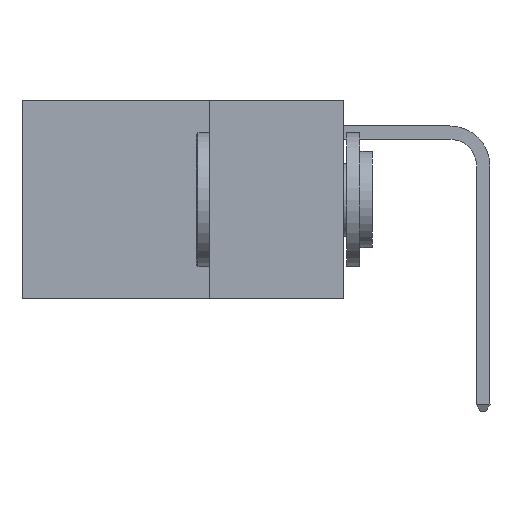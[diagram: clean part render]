
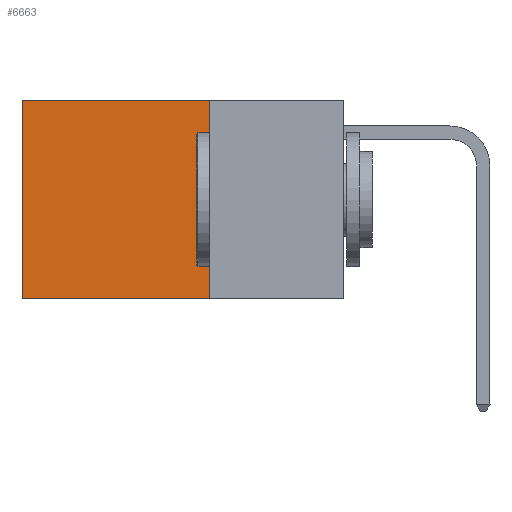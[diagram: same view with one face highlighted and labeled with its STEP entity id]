
A CAD part, left-side view. The second image highlights one B-rep face of the part: STEP entity #6663.
In plain terms, the highlighted planar face has unit normal (-1, 0, 0).
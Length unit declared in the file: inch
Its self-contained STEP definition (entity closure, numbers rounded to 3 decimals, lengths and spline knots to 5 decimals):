
#98 = LINE ( 'NONE', #18927, #11334 ) ;
#818 = CARTESIAN_POINT ( 'NONE',  ( 0.2625, 0.25, 0. ) ) ;
#1428 = EDGE_LOOP ( 'NONE', ( #16039, #3002, #7451, #16599 ) ) ;
#1531 = CARTESIAN_POINT ( 'NONE',  ( 0.2625, 0.6, -0.37 ) ) ;
#1588 = DIRECTION ( 'NONE',  ( 0., 1., 0. ) ) ;
#1598 = DIRECTION ( 'NONE',  ( 0., 0., -1. ) ) ;
#1972 = CARTESIAN_POINT ( 'NONE',  ( 0.2625, 0.6, 0. ) ) ;
#2397 = CARTESIAN_POINT ( 'NONE',  ( 0.2625, 0.6, 0. ) ) ;
#2814 = VERTEX_POINT ( 'NONE', #1531 ) ;
#2885 = DIRECTION ( 'NONE',  ( 0., 1., 0. ) ) ;
#3002 = ORIENTED_EDGE ( 'NONE', *, *, #4521, .F. ) ;
#3308 = LINE ( 'NONE', #9067, #15841 ) ;
#4463 = CARTESIAN_POINT ( 'NONE',  ( 0.2625, 0.25, -0.37 ) ) ;
#4521 = EDGE_CURVE ( 'NONE', #5329, #2814, #98, .T. ) ;
#5253 = DIRECTION ( 'NONE',  ( 0., 0., -1. ) ) ;
#5329 = VERTEX_POINT ( 'NONE', #4463 ) ;
#6663 = ADVANCED_FACE ( 'NONE', ( #7265 ), #14650, .F. ) ;
#6981 = VERTEX_POINT ( 'NONE', #818 ) ;
#7265 = FACE_OUTER_BOUND ( 'NONE', #1428, .T. ) ;
#7451 = ORIENTED_EDGE ( 'NONE', *, *, #9723, .F. ) ;
#9067 = CARTESIAN_POINT ( 'NONE',  ( 0.2625, 0.25, 0. ) ) ;
#9491 = LINE ( 'NONE', #18412, #13895 ) ;
#9723 = EDGE_CURVE ( 'NONE', #6981, #5329, #9491, .T. ) ;
#11334 = VECTOR ( 'NONE', #2885, 39.37008 ) ;
#11668 = CARTESIAN_POINT ( 'NONE',  ( 0.2625, 0.25, 0. ) ) ;
#13013 = DIRECTION ( 'NONE',  ( 1., 0., 0. ) ) ;
#13579 = EDGE_CURVE ( 'NONE', #6981, #14648, #3308, .T. ) ;
#13657 = DIRECTION ( 'NONE',  ( 0., 0., -1. ) ) ;
#13895 = VECTOR ( 'NONE', #5253, 39.37008 ) ;
#14371 = VECTOR ( 'NONE', #13657, 39.37008 ) ;
#14648 = VERTEX_POINT ( 'NONE', #2397 ) ;
#14650 = PLANE ( 'NONE',  #15455 ) ;
#15107 = LINE ( 'NONE', #1972, #14371 ) ;
#15455 = AXIS2_PLACEMENT_3D ( 'NONE', #11668, #13013, #1598 ) ;
#15841 = VECTOR ( 'NONE', #1588, 39.37008 ) ;
#16039 = ORIENTED_EDGE ( 'NONE', *, *, #18622, .T. ) ;
#16599 = ORIENTED_EDGE ( 'NONE', *, *, #13579, .T. ) ;
#18412 = CARTESIAN_POINT ( 'NONE',  ( 0.2625, 0.25, 0. ) ) ;
#18622 = EDGE_CURVE ( 'NONE', #14648, #2814, #15107, .T. ) ;
#18927 = CARTESIAN_POINT ( 'NONE',  ( 0.2625, 0.25, -0.37 ) ) ;
